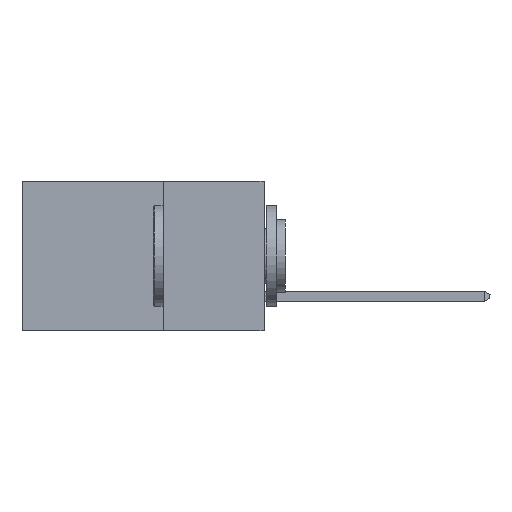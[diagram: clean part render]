
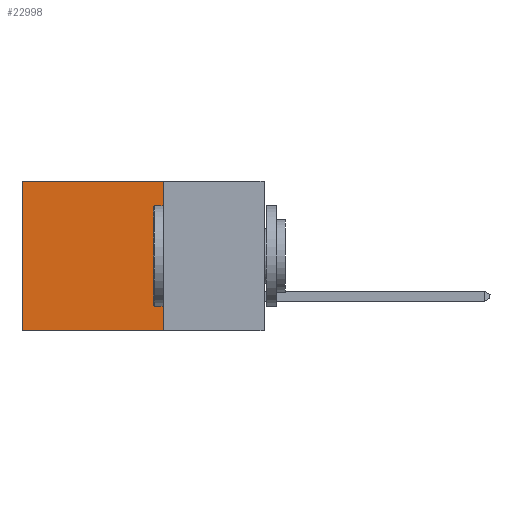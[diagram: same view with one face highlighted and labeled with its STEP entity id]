
A CAD part, left-side view. The second image highlights one B-rep face of the part: STEP entity #22998.
In plain terms, the highlighted planar face has unit normal (-1, 0, 0).
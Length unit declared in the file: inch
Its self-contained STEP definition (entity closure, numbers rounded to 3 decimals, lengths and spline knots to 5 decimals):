
#1665 = CARTESIAN_POINT ( 'NONE',  ( 0.298, 0.6, 0. ) ) ;
#2249 = EDGE_CURVE ( 'NONE', #24162, #22187, #10778, .T. ) ;
#3357 = EDGE_CURVE ( 'NONE', #22187, #14790, #12233, .T. ) ;
#3362 = VERTEX_POINT ( 'NONE', #1665 ) ;
#4142 = EDGE_CURVE ( 'NONE', #3362, #14790, #16296, .T. ) ;
#5119 = ORIENTED_EDGE ( 'NONE', *, *, #4142, .T. ) ;
#5515 = PLANE ( 'NONE',  #22272 ) ;
#5696 = DIRECTION ( 'NONE',  ( 0., 0., -1. ) ) ;
#5962 = CARTESIAN_POINT ( 'NONE',  ( 0.298, 0.6, 0. ) ) ;
#6949 = CARTESIAN_POINT ( 'NONE',  ( 0.298, 0.6, -0.37 ) ) ;
#7008 = ORIENTED_EDGE ( 'NONE', *, *, #11217, .T. ) ;
#7450 = DIRECTION ( 'NONE',  ( 0., 1., 0. ) ) ;
#7511 = DIRECTION ( 'NONE',  ( 1., 0., 0. ) ) ;
#9603 = CARTESIAN_POINT ( 'NONE',  ( 0.298, 0.25, -0.37 ) ) ;
#9705 = LINE ( 'NONE', #18533, #10610 ) ;
#9870 = VECTOR ( 'NONE', #17948, 39.37008 ) ;
#10610 = VECTOR ( 'NONE', #16815, 39.37008 ) ;
#10778 = LINE ( 'NONE', #20085, #9870 ) ;
#11217 = EDGE_CURVE ( 'NONE', #24162, #3362, #9705, .T. ) ;
#12233 = LINE ( 'NONE', #9603, #21077 ) ;
#12790 = EDGE_LOOP ( 'NONE', ( #5119, #23063, #16998, #7008 ) ) ;
#14790 = VERTEX_POINT ( 'NONE', #6949 ) ;
#15586 = CARTESIAN_POINT ( 'NONE',  ( 0.298, 0.25, 0. ) ) ;
#16296 = LINE ( 'NONE', #5962, #19538 ) ;
#16815 = DIRECTION ( 'NONE',  ( 0., 1., 0. ) ) ;
#16998 = ORIENTED_EDGE ( 'NONE', *, *, #2249, .F. ) ;
#17163 = DIRECTION ( 'NONE',  ( 0., 0., -1. ) ) ;
#17948 = DIRECTION ( 'NONE',  ( 0., 0., -1. ) ) ;
#18533 = CARTESIAN_POINT ( 'NONE',  ( 0.298, 0.25, 0. ) ) ;
#18902 = CARTESIAN_POINT ( 'NONE',  ( 0.298, 0.25, -0.37 ) ) ;
#19538 = VECTOR ( 'NONE', #17163, 39.37008 ) ;
#20085 = CARTESIAN_POINT ( 'NONE',  ( 0.298, 0.25, 0. ) ) ;
#20702 = CARTESIAN_POINT ( 'NONE',  ( 0.298, 0.25, 0. ) ) ;
#21077 = VECTOR ( 'NONE', #7450, 39.37008 ) ;
#21424 = FACE_OUTER_BOUND ( 'NONE', #12790, .T. ) ;
#22187 = VERTEX_POINT ( 'NONE', #18902 ) ;
#22272 = AXIS2_PLACEMENT_3D ( 'NONE', #20702, #7511, #5696 ) ;
#22998 = ADVANCED_FACE ( 'NONE', ( #21424 ), #5515, .F. ) ;
#23063 = ORIENTED_EDGE ( 'NONE', *, *, #3357, .F. ) ;
#24162 = VERTEX_POINT ( 'NONE', #15586 ) ;
